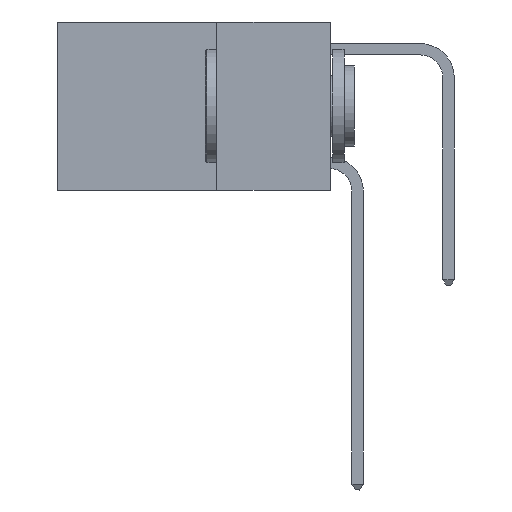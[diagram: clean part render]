
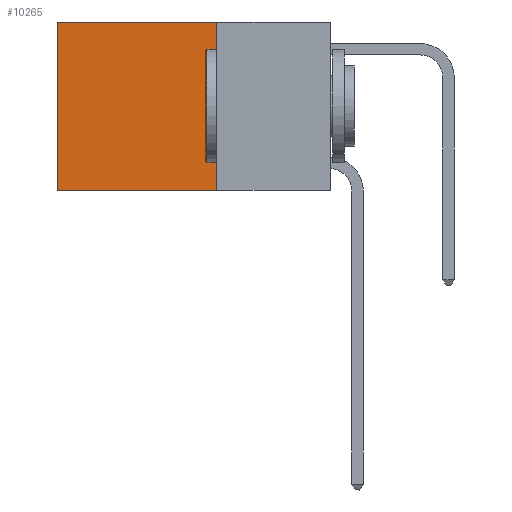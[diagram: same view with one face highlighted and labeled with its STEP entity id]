
A CAD part, left-side view. The second image highlights one B-rep face of the part: STEP entity #10265.
In plain terms, the highlighted planar face has unit normal (-1, 0, 0).
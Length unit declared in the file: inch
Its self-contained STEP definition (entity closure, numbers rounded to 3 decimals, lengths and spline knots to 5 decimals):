
#1046 = ORIENTED_EDGE ( 'NONE', *, *, #18340, .T. ) ;
#1255 = LINE ( 'NONE', #7230, #9783 ) ;
#1736 = PLANE ( 'NONE',  #27032 ) ;
#2375 = CARTESIAN_POINT ( 'NONE',  ( 0.2625, 0.25, -0.37 ) ) ;
#3277 = LINE ( 'NONE', #26658, #16915 ) ;
#4714 = ORIENTED_EDGE ( 'NONE', *, *, #12095, .F. ) ;
#5710 = CARTESIAN_POINT ( 'NONE',  ( 0.2625, 0.6, 0. ) ) ;
#7230 = CARTESIAN_POINT ( 'NONE',  ( 0.2625, 0.6, 0. ) ) ;
#7973 = DIRECTION ( 'NONE',  ( 0., 1., 0. ) ) ;
#9585 = CARTESIAN_POINT ( 'NONE',  ( 0.2625, 0.25, 0. ) ) ;
#9747 = LINE ( 'NONE', #9585, #15189 ) ;
#9783 = VECTOR ( 'NONE', #24838, 39.37008 ) ;
#9981 = EDGE_CURVE ( 'NONE', #16446, #19386, #1255, .T. ) ;
#10004 = VECTOR ( 'NONE', #7973, 39.37008 ) ;
#10265 = ADVANCED_FACE ( 'NONE', ( #24200 ), #1736, .F. ) ;
#12095 = EDGE_CURVE ( 'NONE', #23719, #19386, #14096, .T. ) ;
#14057 = DIRECTION ( 'NONE',  ( 0., 1., 0. ) ) ;
#14096 = LINE ( 'NONE', #16932, #10004 ) ;
#14158 = VERTEX_POINT ( 'NONE', #20711 ) ;
#15189 = VECTOR ( 'NONE', #14057, 39.37008 ) ;
#15504 = ORIENTED_EDGE ( 'NONE', *, *, #18601, .F. ) ;
#16446 = VERTEX_POINT ( 'NONE', #5710 ) ;
#16915 = VECTOR ( 'NONE', #18102, 39.37008 ) ;
#16932 = CARTESIAN_POINT ( 'NONE',  ( 0.2625, 0.25, -0.37 ) ) ;
#16942 = CARTESIAN_POINT ( 'NONE',  ( 0.2625, 0.25, 0. ) ) ;
#18102 = DIRECTION ( 'NONE',  ( 0., 0., -1. ) ) ;
#18340 = EDGE_CURVE ( 'NONE', #14158, #16446, #9747, .T. ) ;
#18601 = EDGE_CURVE ( 'NONE', #14158, #23719, #3277, .T. ) ;
#19386 = VERTEX_POINT ( 'NONE', #20665 ) ;
#20665 = CARTESIAN_POINT ( 'NONE',  ( 0.2625, 0.6, -0.37 ) ) ;
#20711 = CARTESIAN_POINT ( 'NONE',  ( 0.2625, 0.25, 0. ) ) ;
#20859 = EDGE_LOOP ( 'NONE', ( #22547, #4714, #15504, #1046 ) ) ;
#21180 = DIRECTION ( 'NONE',  ( 0., 0., -1. ) ) ;
#21457 = DIRECTION ( 'NONE',  ( 1., 0., 0. ) ) ;
#22547 = ORIENTED_EDGE ( 'NONE', *, *, #9981, .T. ) ;
#23719 = VERTEX_POINT ( 'NONE', #2375 ) ;
#24200 = FACE_OUTER_BOUND ( 'NONE', #20859, .T. ) ;
#24838 = DIRECTION ( 'NONE',  ( 0., 0., -1. ) ) ;
#26658 = CARTESIAN_POINT ( 'NONE',  ( 0.2625, 0.25, 0. ) ) ;
#27032 = AXIS2_PLACEMENT_3D ( 'NONE', #16942, #21457, #21180 ) ;
